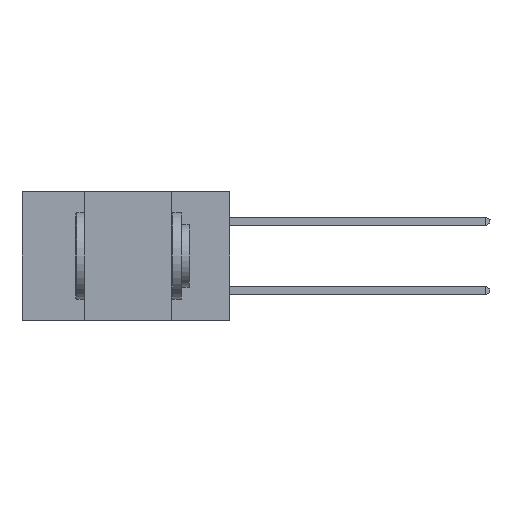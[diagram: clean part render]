
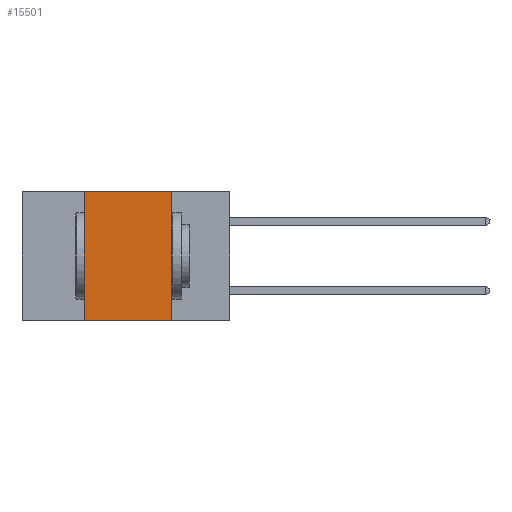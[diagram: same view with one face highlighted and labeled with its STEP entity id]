
A CAD part, left-side view. The second image highlights one B-rep face of the part: STEP entity #15501.
In plain terms, the highlighted planar face has unit normal (-1, 0, 0).
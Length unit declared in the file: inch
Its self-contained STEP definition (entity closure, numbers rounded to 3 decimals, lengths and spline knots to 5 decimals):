
#235 = VECTOR ( 'NONE', #14395, 39.37008 ) ;
#513 = LINE ( 'NONE', #1920, #3465 ) ;
#534 = LINE ( 'NONE', #8911, #12012 ) ;
#805 = VERTEX_POINT ( 'NONE', #3491 ) ;
#1167 = ORIENTED_EDGE ( 'NONE', *, *, #1295, .F. ) ;
#1188 = FACE_OUTER_BOUND ( 'NONE', #4181, .T. ) ;
#1295 = EDGE_CURVE ( 'NONE', #15340, #805, #513, .T. ) ;
#1752 = LINE ( 'NONE', #13639, #14058 ) ;
#1801 = ORIENTED_EDGE ( 'NONE', *, *, #4979, .F. ) ;
#1920 = CARTESIAN_POINT ( 'NONE',  ( 0., 0.17, -0.37 ) ) ;
#2623 = EDGE_CURVE ( 'NONE', #12080, #14066, #534, .T. ) ;
#3465 = VECTOR ( 'NONE', #6710, 39.37008 ) ;
#3491 = CARTESIAN_POINT ( 'NONE',  ( 0., 0.17, -0.37 ) ) ;
#4181 = EDGE_LOOP ( 'NONE', ( #1167, #1801, #10808, #5677 ) ) ;
#4820 = LINE ( 'NONE', #9580, #235 ) ;
#4979 = EDGE_CURVE ( 'NONE', #14066, #15340, #4820, .T. ) ;
#5677 = ORIENTED_EDGE ( 'NONE', *, *, #5972, .T. ) ;
#5906 = DIRECTION ( 'NONE',  ( 1., 0., 0. ) ) ;
#5972 = EDGE_CURVE ( 'NONE', #12080, #805, #1752, .T. ) ;
#5974 = PLANE ( 'NONE',  #9225 ) ;
#6710 = DIRECTION ( 'NONE',  ( 0., 0., -1. ) ) ;
#8911 = CARTESIAN_POINT ( 'NONE',  ( 0., 0.42, -0.37 ) ) ;
#9225 = AXIS2_PLACEMENT_3D ( 'NONE', #10769, #5906, #10692 ) ;
#9580 = CARTESIAN_POINT ( 'NONE',  ( 0., 0.6, 0. ) ) ;
#10692 = DIRECTION ( 'NONE',  ( 0., 0., -1. ) ) ;
#10766 = CARTESIAN_POINT ( 'NONE',  ( 0., 0.42, 0. ) ) ;
#10769 = CARTESIAN_POINT ( 'NONE',  ( 0., 0.6, 0. ) ) ;
#10808 = ORIENTED_EDGE ( 'NONE', *, *, #2623, .F. ) ;
#12012 = VECTOR ( 'NONE', #13738, 39.37008 ) ;
#12080 = VERTEX_POINT ( 'NONE', #14546 ) ;
#13639 = CARTESIAN_POINT ( 'NONE',  ( 0., 0.6, -0.37 ) ) ;
#13709 = CARTESIAN_POINT ( 'NONE',  ( 0., 0.17, 0. ) ) ;
#13738 = DIRECTION ( 'NONE',  ( 0., 0., 1. ) ) ;
#13877 = DIRECTION ( 'NONE',  ( 0., -1., 0. ) ) ;
#14058 = VECTOR ( 'NONE', #13877, 39.37008 ) ;
#14066 = VERTEX_POINT ( 'NONE', #10766 ) ;
#14395 = DIRECTION ( 'NONE',  ( 0., -1., 0. ) ) ;
#14546 = CARTESIAN_POINT ( 'NONE',  ( 0., 0.42, -0.37 ) ) ;
#15340 = VERTEX_POINT ( 'NONE', #13709 ) ;
#15501 = ADVANCED_FACE ( 'NONE', ( #1188 ), #5974, .F. ) ;
